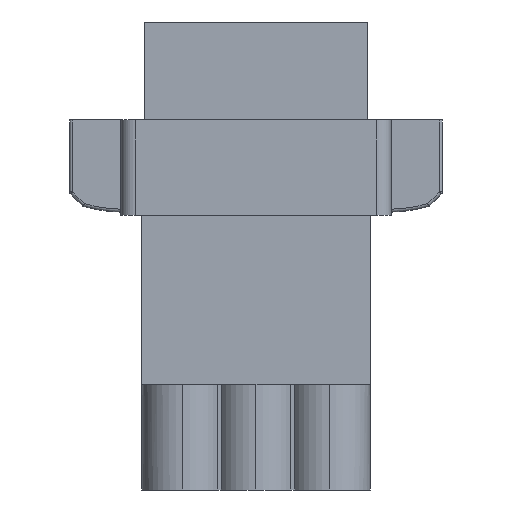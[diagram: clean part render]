
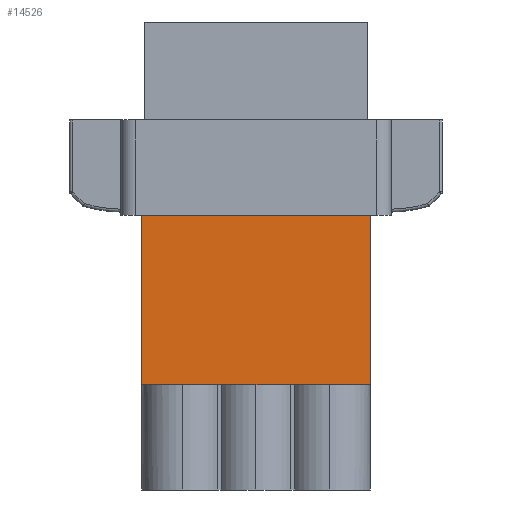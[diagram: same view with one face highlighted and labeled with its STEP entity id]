
A CAD part, front view. The second image highlights one B-rep face of the part: STEP entity #14526.
In plain terms, the highlighted planar face has unit normal (0, -1, 0).
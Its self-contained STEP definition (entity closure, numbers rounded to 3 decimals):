
#796 = VERTEX_POINT ( 'NONE', #11671 ) ;
#1026 = EDGE_LOOP ( 'NONE', ( #5075, #1553, #9309, #5242 ) ) ;
#1553 = ORIENTED_EDGE ( 'NONE', *, *, #15091, .F. ) ;
#2227 = CARTESIAN_POINT ( 'NONE',  ( -7.8, -6.3, -11.6 ) ) ;
#2315 = DIRECTION ( 'NONE',  ( 1., 0., 0. ) ) ;
#2650 = DIRECTION ( 'NONE',  ( 0., 0., 1. ) ) ;
#2677 = VECTOR ( 'NONE', #5805, 1000. ) ;
#3227 = EDGE_CURVE ( 'NONE', #5107, #12410, #10009, .T. ) ;
#3314 = DIRECTION ( 'NONE',  ( 1., 0., 0. ) ) ;
#4710 = CARTESIAN_POINT ( 'NONE',  ( 7.8, -6.3, -11.6 ) ) ;
#4720 = LINE ( 'NONE', #13942, #2677 ) ;
#5075 = ORIENTED_EDGE ( 'NONE', *, *, #12044, .F. ) ;
#5107 = VERTEX_POINT ( 'NONE', #2227 ) ;
#5184 = VECTOR ( 'NONE', #16987, 1000. ) ;
#5242 = ORIENTED_EDGE ( 'NONE', *, *, #9366, .T. ) ;
#5495 = VECTOR ( 'NONE', #2650, 1000. ) ;
#5805 = DIRECTION ( 'NONE',  ( 0., 0., 1. ) ) ;
#6168 = CARTESIAN_POINT ( 'NONE',  ( 0., -6.3, -11.6 ) ) ;
#7609 = PLANE ( 'NONE',  #16616 ) ;
#8759 = CARTESIAN_POINT ( 'NONE',  ( 0., -6.3, 0. ) ) ;
#9173 = CARTESIAN_POINT ( 'NONE',  ( -7.8, -6.3, -11.6 ) ) ;
#9309 = ORIENTED_EDGE ( 'NONE', *, *, #3227, .T. ) ;
#9366 = EDGE_CURVE ( 'NONE', #12410, #796, #4720, .T. ) ;
#10009 = LINE ( 'NONE', #15467, #10303 ) ;
#10303 = VECTOR ( 'NONE', #2315, 1000. ) ;
#10355 = CARTESIAN_POINT ( 'NONE',  ( -7.8, -6.3, 0. ) ) ;
#10905 = VERTEX_POINT ( 'NONE', #10355 ) ;
#11621 = LINE ( 'NONE', #8759, #5184 ) ;
#11671 = CARTESIAN_POINT ( 'NONE',  ( 7.8, -6.3, 0. ) ) ;
#12044 = EDGE_CURVE ( 'NONE', #10905, #796, #11621, .T. ) ;
#12410 = VERTEX_POINT ( 'NONE', #4710 ) ;
#13050 = DIRECTION ( 'NONE',  ( 0., -1., 0. ) ) ;
#13942 = CARTESIAN_POINT ( 'NONE',  ( 7.8, -6.3, -11.6 ) ) ;
#14219 = FACE_OUTER_BOUND ( 'NONE', #1026, .T. ) ;
#14526 = ADVANCED_FACE ( 'NONE', ( #14219 ), #7609, .T. ) ;
#15091 = EDGE_CURVE ( 'NONE', #5107, #10905, #16321, .T. ) ;
#15467 = CARTESIAN_POINT ( 'NONE',  ( 0., -6.3, -11.6 ) ) ;
#16321 = LINE ( 'NONE', #9173, #5495 ) ;
#16616 = AXIS2_PLACEMENT_3D ( 'NONE', #6168, #13050, #3314 ) ;
#16987 = DIRECTION ( 'NONE',  ( 1., 0., 0. ) ) ;
